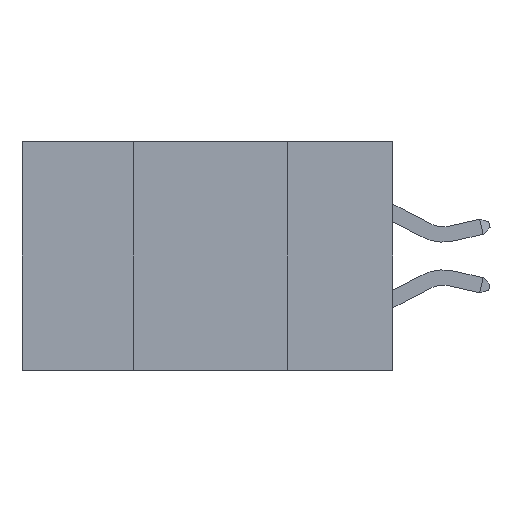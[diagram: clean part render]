
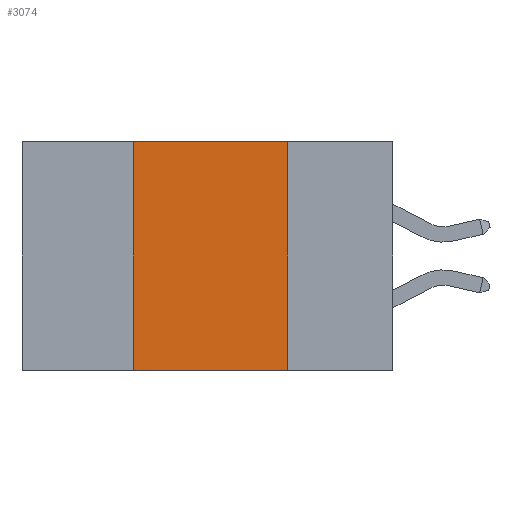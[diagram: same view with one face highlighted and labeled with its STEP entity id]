
A CAD part, left-side view. The second image highlights one B-rep face of the part: STEP entity #3074.
In plain terms, the highlighted planar face has unit normal (-1, 0, 0).
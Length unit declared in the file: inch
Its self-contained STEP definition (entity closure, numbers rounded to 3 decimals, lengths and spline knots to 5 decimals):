
#223 = ORIENTED_EDGE ( 'NONE', *, *, #7124, .F. ) ;
#310 = CARTESIAN_POINT ( 'NONE',  ( 0., 0.17, -0.37 ) ) ;
#1095 = VERTEX_POINT ( 'NONE', #7508 ) ;
#1099 = DIRECTION ( 'NONE',  ( 0., 0., -1. ) ) ;
#1602 = VECTOR ( 'NONE', #2099, 39.37008 ) ;
#1801 = AXIS2_PLACEMENT_3D ( 'NONE', #12124, #4729, #1099 ) ;
#2099 = DIRECTION ( 'NONE',  ( 0., 0., 1. ) ) ;
#2415 = DIRECTION ( 'NONE',  ( 0., 0., -1. ) ) ;
#3074 = ADVANCED_FACE ( 'NONE', ( #14565 ), #10861, .F. ) ;
#3162 = VERTEX_POINT ( 'NONE', #11095 ) ;
#3275 = VERTEX_POINT ( 'NONE', #310 ) ;
#4113 = CARTESIAN_POINT ( 'NONE',  ( 0., 0.6, 0. ) ) ;
#4345 = DIRECTION ( 'NONE',  ( 0., -1., 0. ) ) ;
#4425 = DIRECTION ( 'NONE',  ( 0., -1., 0. ) ) ;
#4729 = DIRECTION ( 'NONE',  ( 1., 0., 0. ) ) ;
#4936 = EDGE_CURVE ( 'NONE', #4966, #3275, #5599, .T. ) ;
#4963 = CARTESIAN_POINT ( 'NONE',  ( 0., 0.42, -0.37 ) ) ;
#4966 = VERTEX_POINT ( 'NONE', #4963 ) ;
#5599 = LINE ( 'NONE', #7003, #14167 ) ;
#6472 = ORIENTED_EDGE ( 'NONE', *, *, #4936, .T. ) ;
#7003 = CARTESIAN_POINT ( 'NONE',  ( 0., 0.6, -0.37 ) ) ;
#7124 = EDGE_CURVE ( 'NONE', #4966, #1095, #7927, .T. ) ;
#7153 = VECTOR ( 'NONE', #4425, 39.37008 ) ;
#7508 = CARTESIAN_POINT ( 'NONE',  ( 0., 0.42, 0. ) ) ;
#7927 = LINE ( 'NONE', #10369, #1602 ) ;
#7985 = EDGE_CURVE ( 'NONE', #1095, #3162, #10333, .T. ) ;
#8240 = LINE ( 'NONE', #10756, #14771 ) ;
#8916 = EDGE_LOOP ( 'NONE', ( #9379, #14072, #223, #6472 ) ) ;
#9379 = ORIENTED_EDGE ( 'NONE', *, *, #11902, .F. ) ;
#10333 = LINE ( 'NONE', #4113, #7153 ) ;
#10369 = CARTESIAN_POINT ( 'NONE',  ( 0., 0.42, 0. ) ) ;
#10756 = CARTESIAN_POINT ( 'NONE',  ( 0., 0.17, 0. ) ) ;
#10861 = PLANE ( 'NONE',  #1801 ) ;
#11095 = CARTESIAN_POINT ( 'NONE',  ( 0., 0.17, 0. ) ) ;
#11902 = EDGE_CURVE ( 'NONE', #3162, #3275, #8240, .T. ) ;
#12124 = CARTESIAN_POINT ( 'NONE',  ( 0., 0.6, 0. ) ) ;
#14072 = ORIENTED_EDGE ( 'NONE', *, *, #7985, .F. ) ;
#14167 = VECTOR ( 'NONE', #4345, 39.37008 ) ;
#14565 = FACE_OUTER_BOUND ( 'NONE', #8916, .T. ) ;
#14771 = VECTOR ( 'NONE', #2415, 39.37008 ) ;
